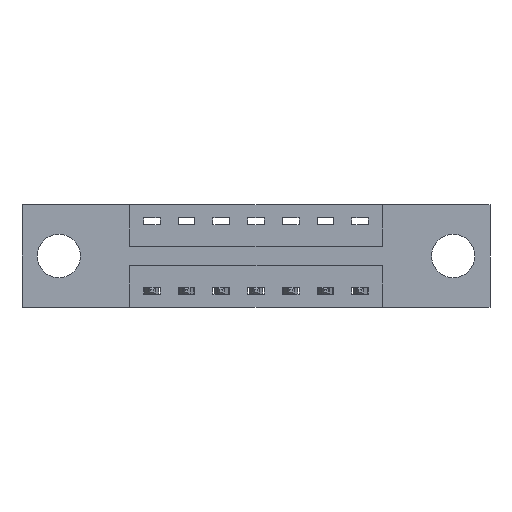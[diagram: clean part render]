
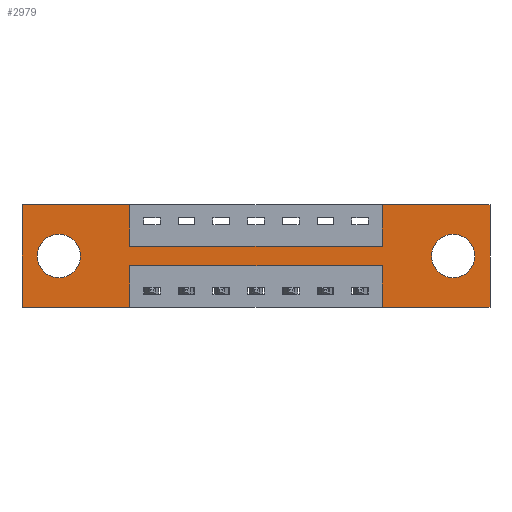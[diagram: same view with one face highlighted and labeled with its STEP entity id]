
A CAD part, front view. The second image highlights one B-rep face of the part: STEP entity #2979.
In plain terms, the highlighted planar face has unit normal (0, -1, 0).
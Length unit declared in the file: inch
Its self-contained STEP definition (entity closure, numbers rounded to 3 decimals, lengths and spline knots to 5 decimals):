
#45 = DIRECTION ( 'NONE',  ( 0., 1., 0. ) ) ;
#95 = EDGE_CURVE ( 'NONE', #3074, #1938, #1347, .T. ) ;
#194 = EDGE_CURVE ( 'NONE', #6700, #6123, #366, .T. ) ;
#366 = LINE ( 'NONE', #1008, #3899 ) ;
#379 = VERTEX_POINT ( 'NONE', #2911 ) ;
#596 = DIRECTION ( 'NONE',  ( 0., 1., 0. ) ) ;
#659 = CIRCLE ( 'NONE', #1457, 0.078 ) ;
#689 = VECTOR ( 'NONE', #795, 39.37008 ) ;
#795 = DIRECTION ( 'NONE',  ( 1., 0., 0. ) ) ;
#846 = ORIENTED_EDGE ( 'NONE', *, *, #4915, .F. ) ;
#880 = DIRECTION ( 'NONE',  ( 0., 0., -1. ) ) ;
#939 = FACE_OUTER_BOUND ( 'NONE', #2420, .T. ) ;
#1008 = CARTESIAN_POINT ( 'NONE',  ( 0., 0., 0. ) ) ;
#1031 = LINE ( 'NONE', #4086, #6155 ) ;
#1059 = VERTEX_POINT ( 'NONE', #4551 ) ;
#1137 = VECTOR ( 'NONE', #7573, 39.37008 ) ;
#1243 = ORIENTED_EDGE ( 'NONE', *, *, #7856, .T. ) ;
#1347 = CIRCLE ( 'NONE', #7759, 0.078 ) ;
#1385 = CARTESIAN_POINT ( 'NONE',  ( 1.2975, 0., -0.22 ) ) ;
#1457 = AXIS2_PLACEMENT_3D ( 'NONE', #2118, #45, #5691 ) ;
#1494 = CARTESIAN_POINT ( 'NONE',  ( 1.685, 0., 0. ) ) ;
#1509 = ORIENTED_EDGE ( 'NONE', *, *, #2453, .F. ) ;
#1606 = VERTEX_POINT ( 'NONE', #7929 ) ;
#1647 = ORIENTED_EDGE ( 'NONE', *, *, #8132, .F. ) ;
#1699 = DIRECTION ( 'NONE',  ( 0., 0., -1. ) ) ;
#1936 = ORIENTED_EDGE ( 'NONE', *, *, #6340, .F. ) ;
#1938 = VERTEX_POINT ( 'NONE', #7177 ) ;
#1948 = ORIENTED_EDGE ( 'NONE', *, *, #3862, .F. ) ;
#2037 = CARTESIAN_POINT ( 'NONE',  ( 0.3875, 0., -0.37 ) ) ;
#2118 = CARTESIAN_POINT ( 'NONE',  ( 1.5525, 0., -0.185 ) ) ;
#2164 = CARTESIAN_POINT ( 'NONE',  ( 0.1325, 0., -0.107 ) ) ;
#2204 = CARTESIAN_POINT ( 'NONE',  ( 0.1325, 0., -0.185 ) ) ;
#2238 = DIRECTION ( 'NONE',  ( 0., 0., -1. ) ) ;
#2243 = CARTESIAN_POINT ( 'NONE',  ( 0.3875, 0., -0.15 ) ) ;
#2297 = DIRECTION ( 'NONE',  ( -1., 0., 0. ) ) ;
#2328 = CARTESIAN_POINT ( 'NONE',  ( 0., 0., -0.37 ) ) ;
#2420 = EDGE_LOOP ( 'NONE', ( #5441, #9030, #1647, #1509, #8729, #3731, #1936, #2505, #846, #6353, #2540, #1948 ) ) ;
#2453 = EDGE_CURVE ( 'NONE', #5846, #379, #1031, .T. ) ;
#2459 = DIRECTION ( 'NONE',  ( 0., 0., 1. ) ) ;
#2480 = CARTESIAN_POINT ( 'NONE',  ( 1.5525, 0., -0.185 ) ) ;
#2505 = ORIENTED_EDGE ( 'NONE', *, *, #3348, .F. ) ;
#2540 = ORIENTED_EDGE ( 'NONE', *, *, #6153, .F. ) ;
#2627 = FACE_BOUND ( 'NONE', #3165, .T. ) ;
#2767 = DIRECTION ( 'NONE',  ( 0., 0., 1. ) ) ;
#2830 = LINE ( 'NONE', #3137, #5909 ) ;
#2867 = PLANE ( 'NONE',  #5202 ) ;
#2911 = CARTESIAN_POINT ( 'NONE',  ( 1.2975, 0., -0.37 ) ) ;
#2979 = ADVANCED_FACE ( 'NONE', ( #4141, #2627, #939 ), #2867, .T. ) ;
#3025 = CARTESIAN_POINT ( 'NONE',  ( 0., 0., 0. ) ) ;
#3033 = VECTOR ( 'NONE', #880, 39.37008 ) ;
#3035 = EDGE_CURVE ( 'NONE', #1059, #8015, #7974, .T. ) ;
#3074 = VERTEX_POINT ( 'NONE', #6717 ) ;
#3137 = CARTESIAN_POINT ( 'NONE',  ( 1.2975, 0., -0.37 ) ) ;
#3151 = VERTEX_POINT ( 'NONE', #1385 ) ;
#3165 = EDGE_LOOP ( 'NONE', ( #6965, #1243 ) ) ;
#3242 = CARTESIAN_POINT ( 'NONE',  ( 1.2975, 0., 0. ) ) ;
#3348 = EDGE_CURVE ( 'NONE', #6536, #4323, #8560, .T. ) ;
#3415 = CARTESIAN_POINT ( 'NONE',  ( 0., 0., 0. ) ) ;
#3436 = EDGE_LOOP ( 'NONE', ( #3705, #8025 ) ) ;
#3453 = EDGE_CURVE ( 'NONE', #3151, #5592, #8042, .T. ) ;
#3705 = ORIENTED_EDGE ( 'NONE', *, *, #4857, .T. ) ;
#3706 = CARTESIAN_POINT ( 'NONE',  ( 0.3875, 0., -0.37 ) ) ;
#3731 = ORIENTED_EDGE ( 'NONE', *, *, #194, .F. ) ;
#3748 = LINE ( 'NONE', #5393, #8209 ) ;
#3827 = DIRECTION ( 'NONE',  ( 0., 1., 0. ) ) ;
#3854 = LINE ( 'NONE', #2328, #8744 ) ;
#3862 = EDGE_CURVE ( 'NONE', #7047, #8508, #3854, .T. ) ;
#3899 = VECTOR ( 'NONE', #5455, 39.37008 ) ;
#3929 = VECTOR ( 'NONE', #7968, 39.37008 ) ;
#4028 = CARTESIAN_POINT ( 'NONE',  ( 0.3875, 0., 0. ) ) ;
#4086 = CARTESIAN_POINT ( 'NONE',  ( 0., 0., -0.37 ) ) ;
#4105 = VERTEX_POINT ( 'NONE', #2164 ) ;
#4141 = FACE_BOUND ( 'NONE', #3436, .T. ) ;
#4270 = CARTESIAN_POINT ( 'NONE',  ( 0., 0., -0.37 ) ) ;
#4323 = VERTEX_POINT ( 'NONE', #7742 ) ;
#4361 = DIRECTION ( 'NONE',  ( 0., -1., 0. ) ) ;
#4551 = CARTESIAN_POINT ( 'NONE',  ( 0., 0., 0. ) ) ;
#4710 = DIRECTION ( 'NONE',  ( 0., 0., 1. ) ) ;
#4855 = EDGE_CURVE ( 'NONE', #4105, #1606, #6779, .T. ) ;
#4857 = EDGE_CURVE ( 'NONE', #1938, #3074, #659, .T. ) ;
#4915 = EDGE_CURVE ( 'NONE', #8015, #6536, #6002, .T. ) ;
#4968 = DIRECTION ( 'NONE',  ( 0., 0., -1. ) ) ;
#4984 = CARTESIAN_POINT ( 'NONE',  ( 0.3875, 0., 0. ) ) ;
#5202 = AXIS2_PLACEMENT_3D ( 'NONE', #4270, #4361, #4968 ) ;
#5236 = DIRECTION ( 'NONE',  ( -1., 0., 0. ) ) ;
#5393 = CARTESIAN_POINT ( 'NONE',  ( 1.685, 0., 0. ) ) ;
#5441 = ORIENTED_EDGE ( 'NONE', *, *, #6913, .F. ) ;
#5455 = DIRECTION ( 'NONE',  ( 1., 0., 0. ) ) ;
#5592 = VERTEX_POINT ( 'NONE', #8172 ) ;
#5691 = DIRECTION ( 'NONE',  ( 0., 0., -1. ) ) ;
#5846 = VERTEX_POINT ( 'NONE', #6107 ) ;
#5909 = VECTOR ( 'NONE', #2459, 39.37008 ) ;
#6002 = LINE ( 'NONE', #4028, #3033 ) ;
#6107 = CARTESIAN_POINT ( 'NONE',  ( 1.685, 0., -0.37 ) ) ;
#6123 = VERTEX_POINT ( 'NONE', #1494 ) ;
#6139 = VECTOR ( 'NONE', #7309, 39.37008 ) ;
#6153 = EDGE_CURVE ( 'NONE', #8508, #1059, #6380, .T. ) ;
#6155 = VECTOR ( 'NONE', #7480, 39.37008 ) ;
#6340 = EDGE_CURVE ( 'NONE', #4323, #6700, #8200, .T. ) ;
#6353 = ORIENTED_EDGE ( 'NONE', *, *, #3035, .F. ) ;
#6380 = LINE ( 'NONE', #3415, #6916 ) ;
#6411 = AXIS2_PLACEMENT_3D ( 'NONE', #2204, #8467, #7108 ) ;
#6430 = CARTESIAN_POINT ( 'NONE',  ( 1.2975, 0., 0. ) ) ;
#6536 = VERTEX_POINT ( 'NONE', #7990 ) ;
#6700 = VERTEX_POINT ( 'NONE', #6430 ) ;
#6717 = CARTESIAN_POINT ( 'NONE',  ( 1.5525, 0., -0.263 ) ) ;
#6779 = CIRCLE ( 'NONE', #8966, 0.078 ) ;
#6913 = EDGE_CURVE ( 'NONE', #5592, #7047, #7149, .T. ) ;
#6916 = VECTOR ( 'NONE', #4710, 39.37008 ) ;
#6965 = ORIENTED_EDGE ( 'NONE', *, *, #4855, .T. ) ;
#7040 = CIRCLE ( 'NONE', #6411, 0.078 ) ;
#7047 = VERTEX_POINT ( 'NONE', #3706 ) ;
#7108 = DIRECTION ( 'NONE',  ( 0., 0., 1. ) ) ;
#7110 = CARTESIAN_POINT ( 'NONE',  ( 0.3875, 0., -0.22 ) ) ;
#7149 = LINE ( 'NONE', #2037, #1137 ) ;
#7177 = CARTESIAN_POINT ( 'NONE',  ( 1.5525, 0., -0.107 ) ) ;
#7309 = DIRECTION ( 'NONE',  ( 0., 0., 1. ) ) ;
#7312 = EDGE_CURVE ( 'NONE', #6123, #5846, #3748, .T. ) ;
#7480 = DIRECTION ( 'NONE',  ( -1., 0., 0. ) ) ;
#7573 = DIRECTION ( 'NONE',  ( 0., 0., -1. ) ) ;
#7704 = CARTESIAN_POINT ( 'NONE',  ( 0., 0., -0.37 ) ) ;
#7742 = CARTESIAN_POINT ( 'NONE',  ( 1.2975, 0., -0.15 ) ) ;
#7759 = AXIS2_PLACEMENT_3D ( 'NONE', #2480, #3827, #1699 ) ;
#7856 = EDGE_CURVE ( 'NONE', #1606, #4105, #7040, .T. ) ;
#7929 = CARTESIAN_POINT ( 'NONE',  ( 0.1325, 0., -0.263 ) ) ;
#7968 = DIRECTION ( 'NONE',  ( 1., 0., 0. ) ) ;
#7974 = LINE ( 'NONE', #3025, #3929 ) ;
#7990 = CARTESIAN_POINT ( 'NONE',  ( 0.3875, 0., -0.15 ) ) ;
#8015 = VERTEX_POINT ( 'NONE', #4984 ) ;
#8025 = ORIENTED_EDGE ( 'NONE', *, *, #95, .T. ) ;
#8042 = LINE ( 'NONE', #7110, #8135 ) ;
#8132 = EDGE_CURVE ( 'NONE', #379, #3151, #2830, .T. ) ;
#8135 = VECTOR ( 'NONE', #2297, 39.37008 ) ;
#8172 = CARTESIAN_POINT ( 'NONE',  ( 0.3875, 0., -0.22 ) ) ;
#8200 = LINE ( 'NONE', #3242, #6139 ) ;
#8209 = VECTOR ( 'NONE', #2238, 39.37008 ) ;
#8467 = DIRECTION ( 'NONE',  ( 0., 1., 0. ) ) ;
#8508 = VERTEX_POINT ( 'NONE', #7704 ) ;
#8560 = LINE ( 'NONE', #2243, #689 ) ;
#8729 = ORIENTED_EDGE ( 'NONE', *, *, #7312, .F. ) ;
#8744 = VECTOR ( 'NONE', #5236, 39.37008 ) ;
#8966 = AXIS2_PLACEMENT_3D ( 'NONE', #8973, #596, #2767 ) ;
#8973 = CARTESIAN_POINT ( 'NONE',  ( 0.1325, 0., -0.185 ) ) ;
#9030 = ORIENTED_EDGE ( 'NONE', *, *, #3453, .F. ) ;
